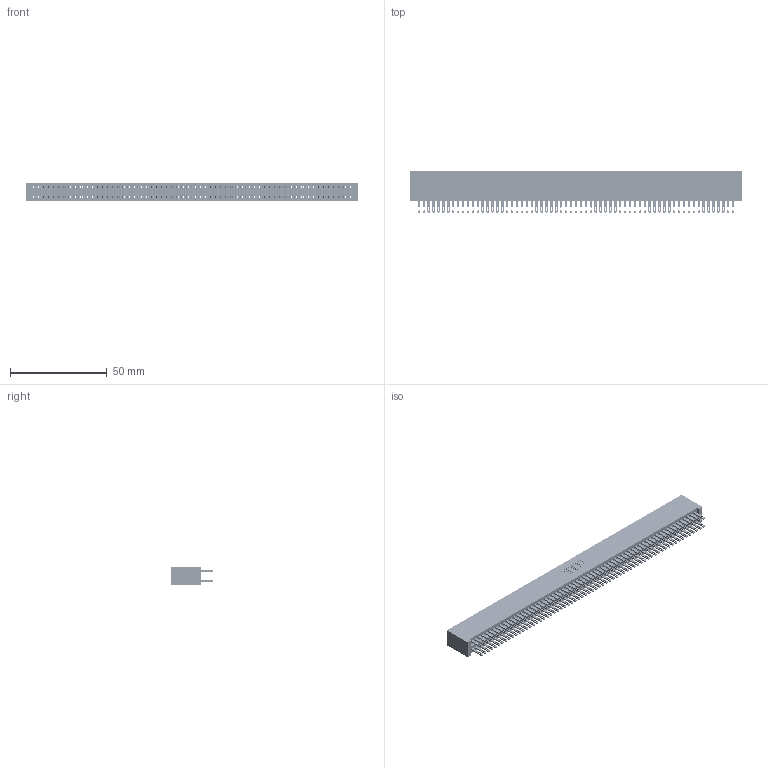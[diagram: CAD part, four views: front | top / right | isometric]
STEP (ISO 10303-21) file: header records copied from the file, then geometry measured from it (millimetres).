
FILE_DESCRIPTION (( 'STEP AP203' ), '1' );
FILE_NAME ('345-130-500-201.STEP', '2019-11-07T11:23:27', ( '' ), ( '' ), 'SwSTEP 2.0', 'SolidWorks 2016', '' );
FILE_SCHEMA (( 'CONFIG_CONTROL_DESIGN' ));
Length unit declared in the file: inch
Products named in the file (3): 345-292-001_345-293-100; 345-130-500-201; 345 Part_No Mounting Lugs
Assembly tree (131 placements, depth 2):
  345-130-500-201
    345 Part_No Mounting Lugs
    345-292-001_345-293-100  x130
Bounding box: 171.7 x 21.51 x 9.4 mm (x, y, z)
Volume: 17906.2 mm3; surface area: 28543 mm2
Topology: 131 solids, 131 shells, 6098 faces, 18647 edges, 12430 vertices
Faces by surface type: plane 3586, cylinder 2512
Entity records: 47557 total; most frequent: CARTESIAN_POINT 7948, ORIENTED_EDGE 7882, DIRECTION 6977, EDGE_CURVE 3941, VECTOR 3553, LINE 3553, VERTEX_POINT 2626, AXIS2_PLACEMENT_3D 1712
